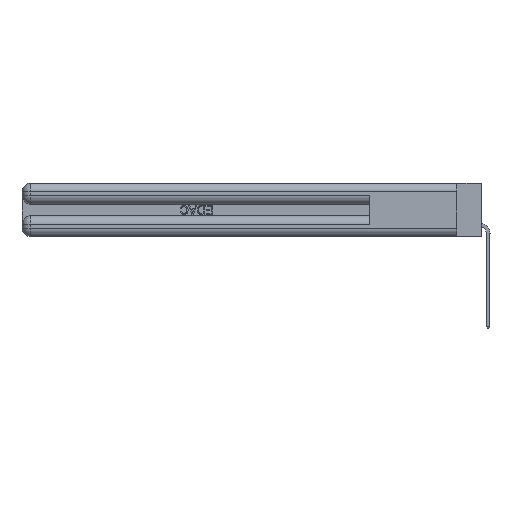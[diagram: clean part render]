
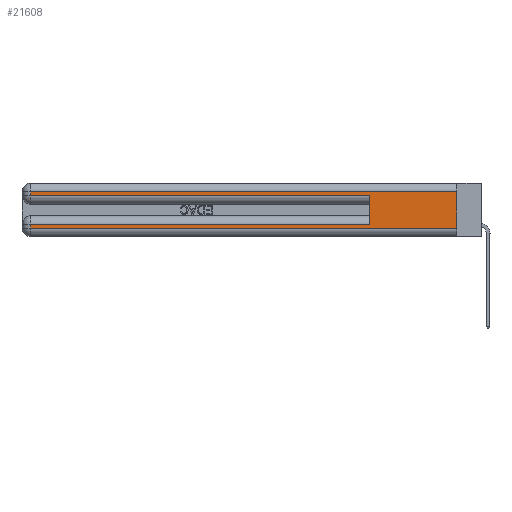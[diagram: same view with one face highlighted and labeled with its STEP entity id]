
A CAD part, left-side view. The second image highlights one B-rep face of the part: STEP entity #21608.
In plain terms, the highlighted planar face has unit normal (-1, 0, 0).
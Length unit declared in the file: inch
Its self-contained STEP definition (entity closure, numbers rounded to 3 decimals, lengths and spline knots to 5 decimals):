
#268 = VERTEX_POINT ( 'NONE', #1283 ) ;
#663 = DIRECTION ( 'NONE',  ( 0., 0., -1. ) ) ;
#746 = VERTEX_POINT ( 'NONE', #8349 ) ;
#1283 = CARTESIAN_POINT ( 'NONE',  ( 0., 0.6, 0.285 ) ) ;
#1399 = LINE ( 'NONE', #9797, #19283 ) ;
#2156 = EDGE_CURVE ( 'NONE', #36530, #16432, #6407, .T. ) ;
#4561 = VECTOR ( 'NONE', #6056, 39.37008 ) ;
#4663 = DIRECTION ( 'NONE',  ( 0., 0., -1. ) ) ;
#4674 = VERTEX_POINT ( 'NONE', #6102 ) ;
#5085 = EDGE_CURVE ( 'NONE', #36530, #268, #7381, .T. ) ;
#5231 = AXIS2_PLACEMENT_3D ( 'NONE', #28055, #42896, #4663 ) ;
#5561 = ORIENTED_EDGE ( 'NONE', *, *, #31923, .F. ) ;
#6056 = DIRECTION ( 'NONE',  ( 0., 1., 0. ) ) ;
#6102 = CARTESIAN_POINT ( 'NONE',  ( 0., 2.94, 0.31 ) ) ;
#6407 = LINE ( 'NONE', #44624, #4561 ) ;
#7381 = LINE ( 'NONE', #30201, #35983 ) ;
#8349 = CARTESIAN_POINT ( 'NONE',  ( 0., 2.94, 0.06 ) ) ;
#8630 = VERTEX_POINT ( 'NONE', #22731 ) ;
#9029 = EDGE_CURVE ( 'NONE', #8630, #4674, #49380, .T. ) ;
#9797 = CARTESIAN_POINT ( 'NONE',  ( 0., 2.94, 0.37 ) ) ;
#9980 = VECTOR ( 'NONE', #37007, 39.37008 ) ;
#12370 = EDGE_CURVE ( 'NONE', #16432, #746, #1399, .T. ) ;
#13483 = VECTOR ( 'NONE', #35900, 39.37008 ) ;
#13625 = CARTESIAN_POINT ( 'NONE',  ( 0., 2.94, 0.285 ) ) ;
#13883 = EDGE_CURVE ( 'NONE', #16954, #268, #45083, .T. ) ;
#16417 = FACE_OUTER_BOUND ( 'NONE', #37769, .T. ) ;
#16432 = VERTEX_POINT ( 'NONE', #45567 ) ;
#16524 = PLANE ( 'NONE',  #5231 ) ;
#16719 = CARTESIAN_POINT ( 'NONE',  ( 0., 0., 0.06 ) ) ;
#16954 = VERTEX_POINT ( 'NONE', #13625 ) ;
#18954 = CARTESIAN_POINT ( 'NONE',  ( 0., 0.6, 0.085 ) ) ;
#19283 = VECTOR ( 'NONE', #44209, 39.37008 ) ;
#19663 = CARTESIAN_POINT ( 'NONE',  ( 0., 0., 0.37 ) ) ;
#21608 = ADVANCED_FACE ( 'NONE', ( #16417 ), #16524, .F. ) ;
#22731 = CARTESIAN_POINT ( 'NONE',  ( 0., 0., 0.31 ) ) ;
#25397 = VECTOR ( 'NONE', #29353, 39.37008 ) ;
#25483 = CARTESIAN_POINT ( 'NONE',  ( 0., 0., 0.285 ) ) ;
#25737 = DIRECTION ( 'NONE',  ( 0., 0., -1. ) ) ;
#26836 = ORIENTED_EDGE ( 'NONE', *, *, #12370, .T. ) ;
#27707 = LINE ( 'NONE', #19663, #42052 ) ;
#28055 = CARTESIAN_POINT ( 'NONE',  ( 0., 0., 0.37 ) ) ;
#29353 = DIRECTION ( 'NONE',  ( 0., -1., 0. ) ) ;
#30201 = CARTESIAN_POINT ( 'NONE',  ( 0., 0.6, 0.145 ) ) ;
#30357 = DIRECTION ( 'NONE',  ( 0., 0., 1. ) ) ;
#31034 = EDGE_CURVE ( 'NONE', #746, #33383, #42673, .T. ) ;
#31923 = EDGE_CURVE ( 'NONE', #8630, #33383, #27707, .T. ) ;
#33265 = ORIENTED_EDGE ( 'NONE', *, *, #5085, .F. ) ;
#33383 = VERTEX_POINT ( 'NONE', #44990 ) ;
#35209 = LINE ( 'NONE', #48718, #44263 ) ;
#35900 = DIRECTION ( 'NONE',  ( 0., -1., 0. ) ) ;
#35983 = VECTOR ( 'NONE', #30357, 39.37008 ) ;
#36530 = VERTEX_POINT ( 'NONE', #18954 ) ;
#37007 = DIRECTION ( 'NONE',  ( 0., 1., 0. ) ) ;
#37769 = EDGE_LOOP ( 'NONE', ( #5561, #42586, #38328, #43442, #33265, #48472, #26836, #44815 ) ) ;
#38328 = ORIENTED_EDGE ( 'NONE', *, *, #40293, .T. ) ;
#40293 = EDGE_CURVE ( 'NONE', #4674, #16954, #35209, .T. ) ;
#42052 = VECTOR ( 'NONE', #663, 39.37008 ) ;
#42586 = ORIENTED_EDGE ( 'NONE', *, *, #9029, .T. ) ;
#42673 = LINE ( 'NONE', #16719, #13483 ) ;
#42896 = DIRECTION ( 'NONE',  ( 1., 0., 0. ) ) ;
#43360 = CARTESIAN_POINT ( 'NONE',  ( 0., 0., 0.31 ) ) ;
#43442 = ORIENTED_EDGE ( 'NONE', *, *, #13883, .T. ) ;
#44209 = DIRECTION ( 'NONE',  ( 0., 0., -1. ) ) ;
#44263 = VECTOR ( 'NONE', #25737, 39.37008 ) ;
#44624 = CARTESIAN_POINT ( 'NONE',  ( 0., 0., 0.085 ) ) ;
#44815 = ORIENTED_EDGE ( 'NONE', *, *, #31034, .T. ) ;
#44990 = CARTESIAN_POINT ( 'NONE',  ( 0., 0., 0.06 ) ) ;
#45083 = LINE ( 'NONE', #25483, #25397 ) ;
#45567 = CARTESIAN_POINT ( 'NONE',  ( 0., 2.94, 0.085 ) ) ;
#48472 = ORIENTED_EDGE ( 'NONE', *, *, #2156, .T. ) ;
#48718 = CARTESIAN_POINT ( 'NONE',  ( 0., 2.94, 0.37 ) ) ;
#49380 = LINE ( 'NONE', #43360, #9980 ) ;
